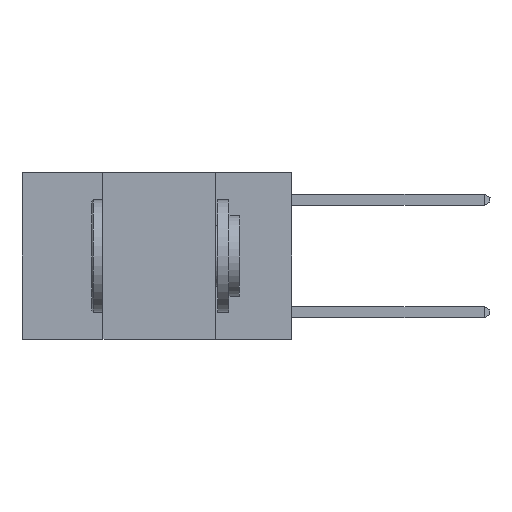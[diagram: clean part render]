
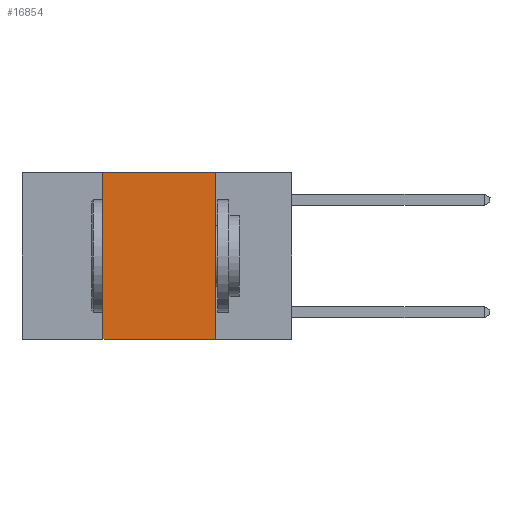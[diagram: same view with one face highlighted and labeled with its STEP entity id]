
A CAD part, left-side view. The second image highlights one B-rep face of the part: STEP entity #16854.
In plain terms, the highlighted planar face has unit normal (-1, 0, 0).
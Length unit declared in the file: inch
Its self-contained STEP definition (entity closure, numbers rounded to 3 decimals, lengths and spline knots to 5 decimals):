
#1558 = DIRECTION ( 'NONE',  ( 0., -1., 0. ) ) ;
#1893 = DIRECTION ( 'NONE',  ( 0., 0., -1. ) ) ;
#2294 = FACE_OUTER_BOUND ( 'NONE', #4102, .T. ) ;
#2680 = DIRECTION ( 'NONE',  ( 0., -1., 0. ) ) ;
#3128 = CARTESIAN_POINT ( 'NONE',  ( 0., 0.6, 0. ) ) ;
#4102 = EDGE_LOOP ( 'NONE', ( #10798, #18831, #12795, #8580 ) ) ;
#4257 = VERTEX_POINT ( 'NONE', #18937 ) ;
#5379 = DIRECTION ( 'NONE',  ( 0., 0., -1. ) ) ;
#6367 = CARTESIAN_POINT ( 'NONE',  ( 0., 0.42, 0. ) ) ;
#6578 = CARTESIAN_POINT ( 'NONE',  ( 0., 0.6, 0. ) ) ;
#6661 = CARTESIAN_POINT ( 'NONE',  ( 0., 0.17, 0. ) ) ;
#7424 = LINE ( 'NONE', #3128, #10388 ) ;
#8353 = DIRECTION ( 'NONE',  ( 0., 0., 1. ) ) ;
#8580 = ORIENTED_EDGE ( 'NONE', *, *, #15183, .T. ) ;
#10388 = VECTOR ( 'NONE', #1558, 39.37008 ) ;
#10674 = CARTESIAN_POINT ( 'NONE',  ( 0., 0.17, -0.37 ) ) ;
#10798 = ORIENTED_EDGE ( 'NONE', *, *, #14310, .F. ) ;
#11095 = PLANE ( 'NONE',  #18347 ) ;
#11546 = LINE ( 'NONE', #6661, #13234 ) ;
#11570 = CARTESIAN_POINT ( 'NONE',  ( 0., 0.6, -0.37 ) ) ;
#12567 = EDGE_CURVE ( 'NONE', #4257, #18787, #12744, .T. ) ;
#12672 = EDGE_CURVE ( 'NONE', #18787, #17485, #7424, .T. ) ;
#12744 = LINE ( 'NONE', #18714, #17248 ) ;
#12795 = ORIENTED_EDGE ( 'NONE', *, *, #12567, .F. ) ;
#12810 = CARTESIAN_POINT ( 'NONE',  ( 0., 0.17, 0. ) ) ;
#13234 = VECTOR ( 'NONE', #5379, 39.37008 ) ;
#14310 = EDGE_CURVE ( 'NONE', #17485, #16019, #11546, .T. ) ;
#14618 = VECTOR ( 'NONE', #2680, 39.37008 ) ;
#15183 = EDGE_CURVE ( 'NONE', #4257, #16019, #18720, .T. ) ;
#16019 = VERTEX_POINT ( 'NONE', #10674 ) ;
#16854 = ADVANCED_FACE ( 'NONE', ( #2294 ), #11095, .F. ) ;
#17238 = DIRECTION ( 'NONE',  ( 1., 0., 0. ) ) ;
#17248 = VECTOR ( 'NONE', #8353, 39.37008 ) ;
#17485 = VERTEX_POINT ( 'NONE', #12810 ) ;
#18347 = AXIS2_PLACEMENT_3D ( 'NONE', #6578, #17238, #1893 ) ;
#18714 = CARTESIAN_POINT ( 'NONE',  ( 0., 0.42, 0. ) ) ;
#18720 = LINE ( 'NONE', #11570, #14618 ) ;
#18787 = VERTEX_POINT ( 'NONE', #6367 ) ;
#18831 = ORIENTED_EDGE ( 'NONE', *, *, #12672, .F. ) ;
#18937 = CARTESIAN_POINT ( 'NONE',  ( 0., 0.42, -0.37 ) ) ;
